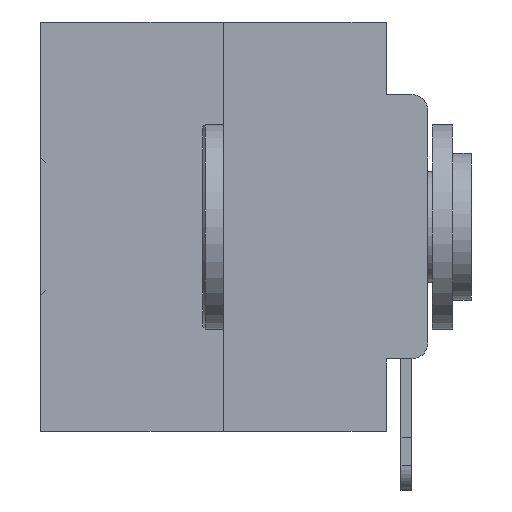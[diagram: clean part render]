
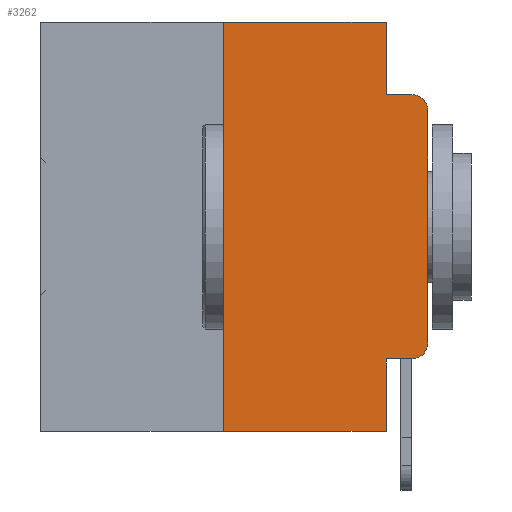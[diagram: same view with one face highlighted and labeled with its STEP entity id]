
A CAD part, left-side view. The second image highlights one B-rep face of the part: STEP entity #3262.
In plain terms, the highlighted planar face has unit normal (-1, 0, 0).
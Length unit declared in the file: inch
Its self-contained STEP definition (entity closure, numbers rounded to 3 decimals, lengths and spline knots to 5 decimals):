
#69 = FACE_OUTER_BOUND ( 'NONE', #32444, .T. ) ;
#412 = VERTEX_POINT ( 'NONE', #33623 ) ;
#467 = ORIENTED_EDGE ( 'NONE', *, *, #2549, .F. ) ;
#583 = ORIENTED_EDGE ( 'NONE', *, *, #624, .T. ) ;
#624 = EDGE_CURVE ( 'NONE', #25400, #4730, #8961, .T. ) ;
#659 = ORIENTED_EDGE ( 'NONE', *, *, #24892, .T. ) ;
#1186 = CARTESIAN_POINT ( 'NONE',  ( 0., 0.02, -0.0885 ) ) ;
#1750 = LINE ( 'NONE', #33586, #8213 ) ;
#2007 = CARTESIAN_POINT ( 'NONE',  ( 0., 0.051, -0.4115 ) ) ;
#2090 = VECTOR ( 'NONE', #21312, 39.37008 ) ;
#2406 = LINE ( 'NONE', #11422, #9779 ) ;
#2549 = EDGE_CURVE ( 'NONE', #25400, #26206, #31389, .T. ) ;
#2585 = AXIS2_PLACEMENT_3D ( 'NONE', #26172, #10234, #28895 ) ;
#3262 = ADVANCED_FACE ( 'NONE', ( #69 ), #10321, .F. ) ;
#4450 = EDGE_CURVE ( 'NONE', #10637, #32947, #24266, .T. ) ;
#4730 = VERTEX_POINT ( 'NONE', #11207 ) ;
#4911 = VECTOR ( 'NONE', #29395, 39.37008 ) ;
#5325 = VERTEX_POINT ( 'NONE', #21650 ) ;
#5954 = VECTOR ( 'NONE', #20359, 39.37008 ) ;
#6734 = VERTEX_POINT ( 'NONE', #25295 ) ;
#7358 = CARTESIAN_POINT ( 'NONE',  ( 0., 0.25, 0. ) ) ;
#7822 = CARTESIAN_POINT ( 'NONE',  ( 0., 0.473, -0.5 ) ) ;
#7916 = CIRCLE ( 'NONE', #29327, 0.02 ) ;
#8082 = EDGE_CURVE ( 'NONE', #5325, #6734, #1750, .T. ) ;
#8095 = CARTESIAN_POINT ( 'NONE',  ( 0., 0.051, -0.5 ) ) ;
#8213 = VECTOR ( 'NONE', #19838, 39.37008 ) ;
#8890 = CARTESIAN_POINT ( 'NONE',  ( 0., 0., -0.1085 ) ) ;
#8961 = LINE ( 'NONE', #27576, #2090 ) ;
#9779 = VECTOR ( 'NONE', #22003, 39.37008 ) ;
#10138 = VECTOR ( 'NONE', #29597, 39.37008 ) ;
#10234 = DIRECTION ( 'NONE',  ( -1., 0., 0. ) ) ;
#10321 = PLANE ( 'NONE',  #30186 ) ;
#10637 = VERTEX_POINT ( 'NONE', #19399 ) ;
#11207 = CARTESIAN_POINT ( 'NONE',  ( 0., 0.02, -0.4115 ) ) ;
#11422 = CARTESIAN_POINT ( 'NONE',  ( 0., 0.051, -0.0885 ) ) ;
#12174 = LINE ( 'NONE', #7822, #4911 ) ;
#12989 = DIRECTION ( 'NONE',  ( 1., 0., 0. ) ) ;
#16001 = EDGE_CURVE ( 'NONE', #32947, #5325, #24907, .T. ) ;
#16138 = DIRECTION ( 'NONE',  ( -1., 0., 0. ) ) ;
#16235 = CARTESIAN_POINT ( 'NONE',  ( 0., 0.25, 0. ) ) ;
#18695 = EDGE_CURVE ( 'NONE', #10637, #26206, #12174, .T. ) ;
#18919 = EDGE_CURVE ( 'NONE', #6734, #28356, #2406, .T. ) ;
#19399 = CARTESIAN_POINT ( 'NONE',  ( 0., 0.25, -0.5 ) ) ;
#19682 = CARTESIAN_POINT ( 'NONE',  ( 0., 0.051, 0. ) ) ;
#19838 = DIRECTION ( 'NONE',  ( 0., 0., -1. ) ) ;
#20359 = DIRECTION ( 'NONE',  ( 0., 0., 1. ) ) ;
#20705 = EDGE_CURVE ( 'NONE', #22282, #28356, #31713, .T. ) ;
#21312 = DIRECTION ( 'NONE',  ( 0., -1., 0. ) ) ;
#21650 = CARTESIAN_POINT ( 'NONE',  ( 0., 0.051, 0. ) ) ;
#22003 = DIRECTION ( 'NONE',  ( 0., -1., 0. ) ) ;
#22282 = VERTEX_POINT ( 'NONE', #8890 ) ;
#22471 = EDGE_CURVE ( 'NONE', #412, #22282, #27391, .T. ) ;
#24071 = VECTOR ( 'NONE', #32694, 39.37008 ) ;
#24266 = LINE ( 'NONE', #16235, #10138 ) ;
#24288 = VECTOR ( 'NONE', #24968, 39.37008 ) ;
#24892 = EDGE_CURVE ( 'NONE', #4730, #412, #7916, .T. ) ;
#24907 = LINE ( 'NONE', #30114, #24071 ) ;
#24968 = DIRECTION ( 'NONE',  ( 0., 0., -1. ) ) ;
#25295 = CARTESIAN_POINT ( 'NONE',  ( 0., 0.051, -0.0885 ) ) ;
#25400 = VERTEX_POINT ( 'NONE', #2007 ) ;
#25774 = ORIENTED_EDGE ( 'NONE', *, *, #22471, .T. ) ;
#25861 = ORIENTED_EDGE ( 'NONE', *, *, #20705, .T. ) ;
#26172 = CARTESIAN_POINT ( 'NONE',  ( 0., 0.02, -0.1085 ) ) ;
#26206 = VERTEX_POINT ( 'NONE', #8095 ) ;
#26449 = ORIENTED_EDGE ( 'NONE', *, *, #18919, .F. ) ;
#27391 = LINE ( 'NONE', #28418, #5954 ) ;
#27392 = ORIENTED_EDGE ( 'NONE', *, *, #8082, .F. ) ;
#27489 = ORIENTED_EDGE ( 'NONE', *, *, #16001, .F. ) ;
#27576 = CARTESIAN_POINT ( 'NONE',  ( 0., 0.051, -0.4115 ) ) ;
#27578 = ORIENTED_EDGE ( 'NONE', *, *, #4450, .F. ) ;
#28356 = VERTEX_POINT ( 'NONE', #1186 ) ;
#28418 = CARTESIAN_POINT ( 'NONE',  ( 0., 0., 0. ) ) ;
#28895 = DIRECTION ( 'NONE',  ( 0., 0., -1. ) ) ;
#28990 = CARTESIAN_POINT ( 'NONE',  ( 0., 0.473, 0. ) ) ;
#29327 = AXIS2_PLACEMENT_3D ( 'NONE', #32127, #16138, #34743 ) ;
#29395 = DIRECTION ( 'NONE',  ( 0., -1., 0. ) ) ;
#29597 = DIRECTION ( 'NONE',  ( 0., 0., 1. ) ) ;
#30114 = CARTESIAN_POINT ( 'NONE',  ( 0., 0.473, 0. ) ) ;
#30186 = AXIS2_PLACEMENT_3D ( 'NONE', #28990, #12989, #31591 ) ;
#31389 = LINE ( 'NONE', #19682, #24288 ) ;
#31591 = DIRECTION ( 'NONE',  ( 0., 0., -1. ) ) ;
#31713 = CIRCLE ( 'NONE', #2585, 0.02 ) ;
#32127 = CARTESIAN_POINT ( 'NONE',  ( 0., 0.02, -0.3915 ) ) ;
#32444 = EDGE_LOOP ( 'NONE', ( #25774, #25861, #26449, #27392, #27489, #27578, #34885, #467, #583, #659 ) ) ;
#32694 = DIRECTION ( 'NONE',  ( 0., -1., 0. ) ) ;
#32947 = VERTEX_POINT ( 'NONE', #7358 ) ;
#33586 = CARTESIAN_POINT ( 'NONE',  ( 0., 0.051, 0. ) ) ;
#33623 = CARTESIAN_POINT ( 'NONE',  ( 0., 0., -0.3915 ) ) ;
#34743 = DIRECTION ( 'NONE',  ( 0., 0., -1. ) ) ;
#34885 = ORIENTED_EDGE ( 'NONE', *, *, #18695, .T. ) ;
